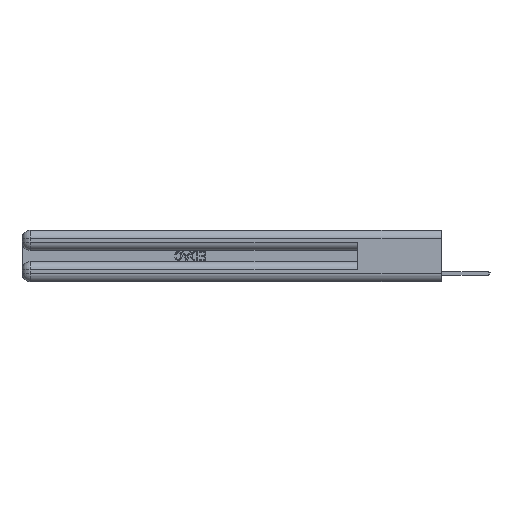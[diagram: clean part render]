
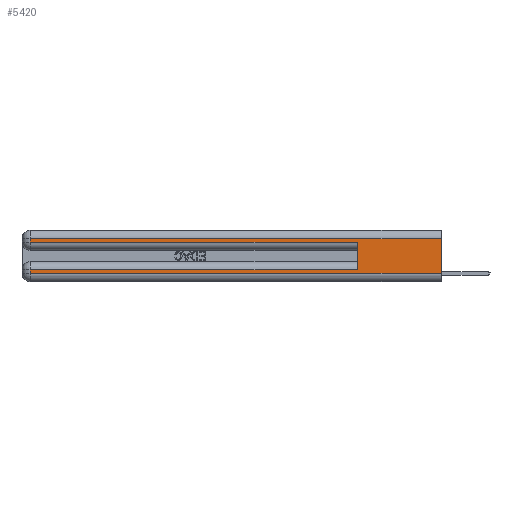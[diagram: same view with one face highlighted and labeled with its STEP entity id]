
A CAD part, left-side view. The second image highlights one B-rep face of the part: STEP entity #5420.
In plain terms, the highlighted planar face has unit normal (-1, 0, 0).
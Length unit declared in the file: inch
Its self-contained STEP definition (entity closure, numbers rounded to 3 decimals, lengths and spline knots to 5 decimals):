
#504 = VERTEX_POINT ( 'NONE', #25668 ) ;
#617 = EDGE_CURVE ( 'NONE', #22041, #11113, #25365, .T. ) ;
#1541 = DIRECTION ( 'NONE',  ( 1., 0., 0. ) ) ;
#1970 = DIRECTION ( 'NONE',  ( 0., 1., 0. ) ) ;
#1993 = CARTESIAN_POINT ( 'NONE',  ( 0., 0., 0.37 ) ) ;
#2160 = CARTESIAN_POINT ( 'NONE',  ( 0., 0., 0.085 ) ) ;
#3931 = AXIS2_PLACEMENT_3D ( 'NONE', #16486, #1541, #14245 ) ;
#4248 = CARTESIAN_POINT ( 'NONE',  ( 0., 2.94, 0.285 ) ) ;
#4505 = CARTESIAN_POINT ( 'NONE',  ( 0., 2.94, 0.06 ) ) ;
#5420 = ADVANCED_FACE ( 'NONE', ( #11258 ), #20781, .F. ) ;
#5770 = VECTOR ( 'NONE', #20938, 39.37008 ) ;
#5996 = VECTOR ( 'NONE', #12017, 39.37008 ) ;
#6128 = VERTEX_POINT ( 'NONE', #25978 ) ;
#8712 = DIRECTION ( 'NONE',  ( 0., 0., -1. ) ) ;
#9161 = EDGE_CURVE ( 'NONE', #504, #6128, #20145, .T. ) ;
#9229 = EDGE_CURVE ( 'NONE', #6128, #16317, #12385, .T. ) ;
#10059 = VECTOR ( 'NONE', #25835, 39.37008 ) ;
#10200 = ORIENTED_EDGE ( 'NONE', *, *, #11529, .T. ) ;
#10618 = CARTESIAN_POINT ( 'NONE',  ( 0., 0., 0.06 ) ) ;
#11067 = CARTESIAN_POINT ( 'NONE',  ( 0., 0., 0.06 ) ) ;
#11113 = VERTEX_POINT ( 'NONE', #13502 ) ;
#11258 = FACE_OUTER_BOUND ( 'NONE', #21403, .T. ) ;
#11529 = EDGE_CURVE ( 'NONE', #11113, #22599, #26230, .T. ) ;
#11945 = ORIENTED_EDGE ( 'NONE', *, *, #617, .T. ) ;
#12017 = DIRECTION ( 'NONE',  ( 0., 1., 0. ) ) ;
#12288 = LINE ( 'NONE', #1993, #23059 ) ;
#12385 = LINE ( 'NONE', #26122, #10059 ) ;
#12781 = ORIENTED_EDGE ( 'NONE', *, *, #26892, .F. ) ;
#13367 = EDGE_CURVE ( 'NONE', #504, #17166, #12288, .T. ) ;
#13502 = CARTESIAN_POINT ( 'NONE',  ( 0., 2.94, 0.085 ) ) ;
#14245 = DIRECTION ( 'NONE',  ( 0., 0., -1. ) ) ;
#14909 = CARTESIAN_POINT ( 'NONE',  ( 0., 0.6, 0.145 ) ) ;
#15664 = VECTOR ( 'NONE', #19880, 39.37008 ) ;
#15826 = ORIENTED_EDGE ( 'NONE', *, *, #21604, .T. ) ;
#16317 = VERTEX_POINT ( 'NONE', #4248 ) ;
#16486 = CARTESIAN_POINT ( 'NONE',  ( 0., 0., 0.37 ) ) ;
#16760 = ORIENTED_EDGE ( 'NONE', *, *, #9161, .T. ) ;
#17156 = DIRECTION ( 'NONE',  ( 0., 0., 1. ) ) ;
#17166 = VERTEX_POINT ( 'NONE', #10618 ) ;
#17899 = ORIENTED_EDGE ( 'NONE', *, *, #9229, .T. ) ;
#18052 = ORIENTED_EDGE ( 'NONE', *, *, #23987, .T. ) ;
#18718 = CARTESIAN_POINT ( 'NONE',  ( 0., 2.94, 0.37 ) ) ;
#19217 = VERTEX_POINT ( 'NONE', #24743 ) ;
#19880 = DIRECTION ( 'NONE',  ( 0., -1., 0. ) ) ;
#20145 = LINE ( 'NONE', #21031, #5996 ) ;
#20295 = VECTOR ( 'NONE', #1970, 39.37008 ) ;
#20765 = DIRECTION ( 'NONE',  ( 0., 0., -1. ) ) ;
#20781 = PLANE ( 'NONE',  #3931 ) ;
#20938 = DIRECTION ( 'NONE',  ( 0., -1., 0. ) ) ;
#21031 = CARTESIAN_POINT ( 'NONE',  ( 0., 0., 0.31 ) ) ;
#21403 = EDGE_LOOP ( 'NONE', ( #21714, #16760, #17899, #18052, #12781, #11945, #10200, #15826 ) ) ;
#21465 = VECTOR ( 'NONE', #17156, 39.37008 ) ;
#21604 = EDGE_CURVE ( 'NONE', #22599, #17166, #27123, .T. ) ;
#21714 = ORIENTED_EDGE ( 'NONE', *, *, #13367, .F. ) ;
#22041 = VERTEX_POINT ( 'NONE', #27781 ) ;
#22599 = VERTEX_POINT ( 'NONE', #4505 ) ;
#23059 = VECTOR ( 'NONE', #8712, 39.37008 ) ;
#23521 = VECTOR ( 'NONE', #20765, 39.37008 ) ;
#23987 = EDGE_CURVE ( 'NONE', #16317, #19217, #24986, .T. ) ;
#24743 = CARTESIAN_POINT ( 'NONE',  ( 0., 0.6, 0.285 ) ) ;
#24986 = LINE ( 'NONE', #27356, #5770 ) ;
#25365 = LINE ( 'NONE', #2160, #20295 ) ;
#25668 = CARTESIAN_POINT ( 'NONE',  ( 0., 0., 0.31 ) ) ;
#25835 = DIRECTION ( 'NONE',  ( 0., 0., -1. ) ) ;
#25978 = CARTESIAN_POINT ( 'NONE',  ( 0., 2.94, 0.31 ) ) ;
#26122 = CARTESIAN_POINT ( 'NONE',  ( 0., 2.94, 0.37 ) ) ;
#26230 = LINE ( 'NONE', #18718, #23521 ) ;
#26892 = EDGE_CURVE ( 'NONE', #22041, #19217, #27208, .T. ) ;
#27123 = LINE ( 'NONE', #11067, #15664 ) ;
#27208 = LINE ( 'NONE', #14909, #21465 ) ;
#27356 = CARTESIAN_POINT ( 'NONE',  ( 0., 0., 0.285 ) ) ;
#27781 = CARTESIAN_POINT ( 'NONE',  ( 0., 0.6, 0.085 ) ) ;
